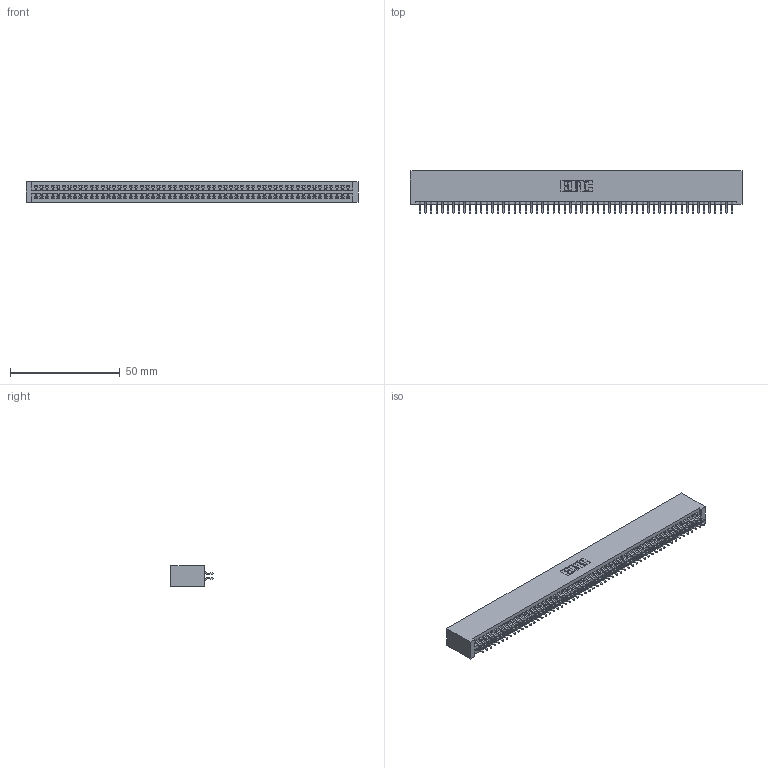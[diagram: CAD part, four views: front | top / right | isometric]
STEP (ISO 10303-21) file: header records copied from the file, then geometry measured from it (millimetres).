
FILE_DESCRIPTION (( 'STEP AP203' ), '1' );
FILE_NAME ('345-114-556-201.STEP', '2018-10-18T15:22:01', ( '' ), ( '' ), 'SwSTEP 2.0', 'SolidWorks 2016', '' );
FILE_SCHEMA (( 'CONFIG_CONTROL_DESIGN' ));
Length unit declared in the file: inch
Products named in the file (3): 345 Part_No Mounting Lugs; 345-292-001_556 Tail; 345-114-556-201
Assembly tree (115 placements, depth 2):
  345-114-556-201
    345 Part_No Mounting Lugs
    345-292-001_556 Tail  x114
Bounding box: 151.38 x 19.24 x 9.4 mm (x, y, z)
Volume: 15456.2 mm3; surface area: 23340.9 mm2
Topology: 115 solids, 115 shells, 6502 faces, 19355 edges, 12750 vertices
Faces by surface type: plane 4294, cylinder 2208
Entity records: 42647 total; most frequent: CARTESIAN_POINT 7148, ORIENTED_EDGE 7070, DIRECTION 6267, EDGE_CURVE 3535, VECTOR 3175, LINE 3175, VERTEX_POINT 2354, AXIS2_PLACEMENT_3D 1546
